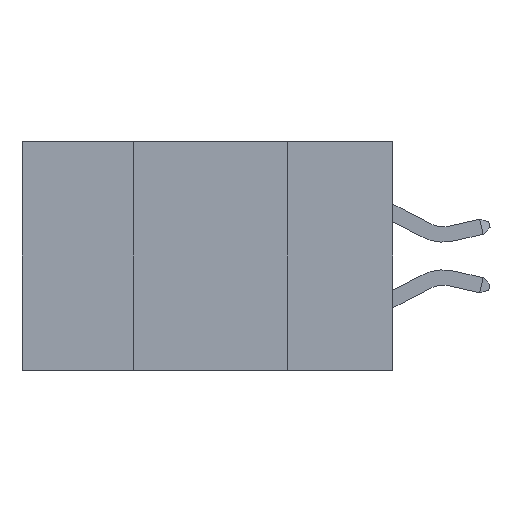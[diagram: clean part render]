
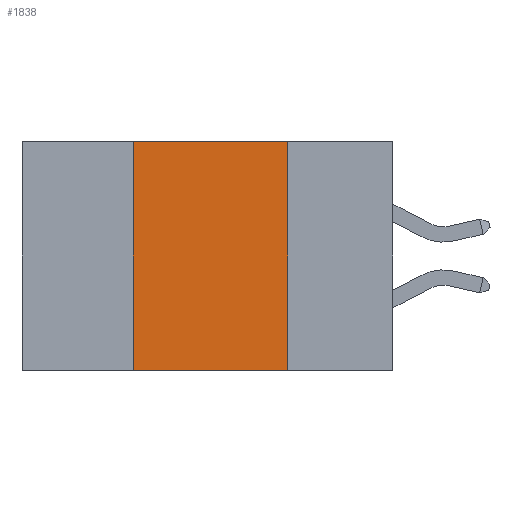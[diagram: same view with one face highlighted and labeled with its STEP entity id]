
A CAD part, left-side view. The second image highlights one B-rep face of the part: STEP entity #1838.
In plain terms, the highlighted planar face has unit normal (-1, 0, 0).
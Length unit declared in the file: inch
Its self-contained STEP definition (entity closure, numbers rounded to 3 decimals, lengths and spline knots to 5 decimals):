
#10 = VERTEX_POINT ( 'NONE', #16828 ) ;
#40 = CARTESIAN_POINT ( 'NONE',  ( 0., 0.6, 0. ) ) ;
#883 = AXIS2_PLACEMENT_3D ( 'NONE', #40, #18359, #8410 ) ;
#1026 = DIRECTION ( 'NONE',  ( 0., 0., 1. ) ) ;
#1772 = FACE_OUTER_BOUND ( 'NONE', #9317, .T. ) ;
#1838 = ADVANCED_FACE ( 'NONE', ( #1772 ), #14982, .F. ) ;
#3141 = ORIENTED_EDGE ( 'NONE', *, *, #6164, .F. ) ;
#4036 = EDGE_CURVE ( 'NONE', #5830, #5067, #9218, .T. ) ;
#5067 = VERTEX_POINT ( 'NONE', #9622 ) ;
#5830 = VERTEX_POINT ( 'NONE', #19069 ) ;
#6164 = EDGE_CURVE ( 'NONE', #12455, #5067, #15914, .T. ) ;
#7952 = DIRECTION ( 'NONE',  ( 0., -1., 0. ) ) ;
#8410 = DIRECTION ( 'NONE',  ( 0., 0., -1. ) ) ;
#8510 = EDGE_CURVE ( 'NONE', #10, #12455, #11168, .T. ) ;
#8800 = DIRECTION ( 'NONE',  ( 0., -1., 0. ) ) ;
#9218 = LINE ( 'NONE', #15387, #16505 ) ;
#9317 = EDGE_LOOP ( 'NONE', ( #3141, #15075, #9381, #19874 ) ) ;
#9381 = ORIENTED_EDGE ( 'NONE', *, *, #10257, .F. ) ;
#9622 = CARTESIAN_POINT ( 'NONE',  ( 0., 0.17, -0.37 ) ) ;
#9886 = CARTESIAN_POINT ( 'NONE',  ( 0., 0.17, 0. ) ) ;
#10257 = EDGE_CURVE ( 'NONE', #5830, #10, #12379, .T. ) ;
#11168 = LINE ( 'NONE', #17908, #20038 ) ;
#11478 = VECTOR ( 'NONE', #21514, 39.37008 ) ;
#12379 = LINE ( 'NONE', #12625, #16823 ) ;
#12455 = VERTEX_POINT ( 'NONE', #14803 ) ;
#12625 = CARTESIAN_POINT ( 'NONE',  ( 0., 0.42, 0. ) ) ;
#14803 = CARTESIAN_POINT ( 'NONE',  ( 0., 0.17, 0. ) ) ;
#14982 = PLANE ( 'NONE',  #883 ) ;
#15075 = ORIENTED_EDGE ( 'NONE', *, *, #8510, .F. ) ;
#15387 = CARTESIAN_POINT ( 'NONE',  ( 0., 0.6, -0.37 ) ) ;
#15914 = LINE ( 'NONE', #9886, #11478 ) ;
#16505 = VECTOR ( 'NONE', #8800, 39.37008 ) ;
#16823 = VECTOR ( 'NONE', #1026, 39.37008 ) ;
#16828 = CARTESIAN_POINT ( 'NONE',  ( 0., 0.42, 0. ) ) ;
#17908 = CARTESIAN_POINT ( 'NONE',  ( 0., 0.6, 0. ) ) ;
#18359 = DIRECTION ( 'NONE',  ( 1., 0., 0. ) ) ;
#19069 = CARTESIAN_POINT ( 'NONE',  ( 0., 0.42, -0.37 ) ) ;
#19874 = ORIENTED_EDGE ( 'NONE', *, *, #4036, .T. ) ;
#20038 = VECTOR ( 'NONE', #7952, 39.37008 ) ;
#21514 = DIRECTION ( 'NONE',  ( 0., 0., -1. ) ) ;
